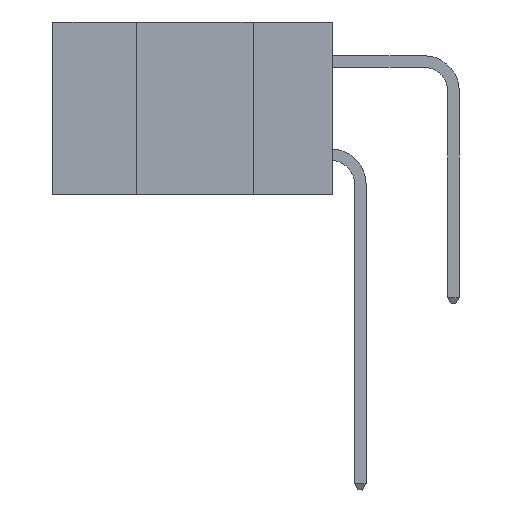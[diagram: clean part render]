
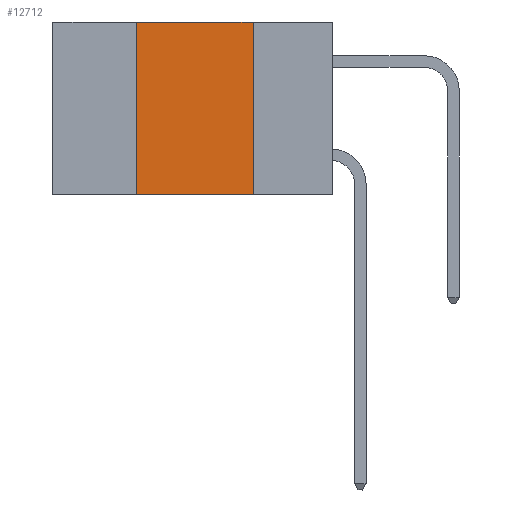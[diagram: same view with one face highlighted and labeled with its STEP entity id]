
A CAD part, left-side view. The second image highlights one B-rep face of the part: STEP entity #12712.
In plain terms, the highlighted planar face has unit normal (-1, 0, 0).
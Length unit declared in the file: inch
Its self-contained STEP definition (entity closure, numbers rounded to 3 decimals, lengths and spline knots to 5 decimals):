
#828 = CARTESIAN_POINT ( 'NONE',  ( 0., 0.17, -0.37 ) ) ;
#1587 = CARTESIAN_POINT ( 'NONE',  ( 0., 0.17, 0. ) ) ;
#2172 = VECTOR ( 'NONE', #2546, 39.37008 ) ;
#2312 = EDGE_CURVE ( 'NONE', #12590, #11486, #14063, .T. ) ;
#2401 = ORIENTED_EDGE ( 'NONE', *, *, #2312, .F. ) ;
#2546 = DIRECTION ( 'NONE',  ( 0., 0., 1. ) ) ;
#2651 = EDGE_CURVE ( 'NONE', #2654, #6762, #3160, .T. ) ;
#2654 = VERTEX_POINT ( 'NONE', #8974 ) ;
#2968 = PLANE ( 'NONE',  #6681 ) ;
#3160 = LINE ( 'NONE', #1587, #13275 ) ;
#4159 = LINE ( 'NONE', #11608, #7142 ) ;
#4472 = CARTESIAN_POINT ( 'NONE',  ( 0., 0.6, 0. ) ) ;
#4949 = ORIENTED_EDGE ( 'NONE', *, *, #8317, .F. ) ;
#5798 = ORIENTED_EDGE ( 'NONE', *, *, #6477, .T. ) ;
#6077 = LINE ( 'NONE', #4472, #11187 ) ;
#6477 = EDGE_CURVE ( 'NONE', #12590, #6762, #4159, .T. ) ;
#6681 = AXIS2_PLACEMENT_3D ( 'NONE', #15557, #15621, #11850 ) ;
#6762 = VERTEX_POINT ( 'NONE', #828 ) ;
#7142 = VECTOR ( 'NONE', #9163, 39.37008 ) ;
#7813 = DIRECTION ( 'NONE',  ( 0., 0., -1. ) ) ;
#8317 = EDGE_CURVE ( 'NONE', #11486, #2654, #6077, .T. ) ;
#8961 = CARTESIAN_POINT ( 'NONE',  ( 0., 0.42, -0.37 ) ) ;
#8974 = CARTESIAN_POINT ( 'NONE',  ( 0., 0.17, 0. ) ) ;
#9089 = ORIENTED_EDGE ( 'NONE', *, *, #2651, .F. ) ;
#9163 = DIRECTION ( 'NONE',  ( 0., -1., 0. ) ) ;
#11187 = VECTOR ( 'NONE', #14601, 39.37008 ) ;
#11486 = VERTEX_POINT ( 'NONE', #15623 ) ;
#11608 = CARTESIAN_POINT ( 'NONE',  ( 0., 0.6, -0.37 ) ) ;
#11850 = DIRECTION ( 'NONE',  ( 0., 0., -1. ) ) ;
#12286 = FACE_OUTER_BOUND ( 'NONE', #13820, .T. ) ;
#12590 = VERTEX_POINT ( 'NONE', #8961 ) ;
#12710 = CARTESIAN_POINT ( 'NONE',  ( 0., 0.42, 0. ) ) ;
#12712 = ADVANCED_FACE ( 'NONE', ( #12286 ), #2968, .F. ) ;
#13275 = VECTOR ( 'NONE', #7813, 39.37008 ) ;
#13820 = EDGE_LOOP ( 'NONE', ( #9089, #4949, #2401, #5798 ) ) ;
#14063 = LINE ( 'NONE', #12710, #2172 ) ;
#14601 = DIRECTION ( 'NONE',  ( 0., -1., 0. ) ) ;
#15557 = CARTESIAN_POINT ( 'NONE',  ( 0., 0.6, 0. ) ) ;
#15621 = DIRECTION ( 'NONE',  ( 1., 0., 0. ) ) ;
#15623 = CARTESIAN_POINT ( 'NONE',  ( 0., 0.42, 0. ) ) ;
